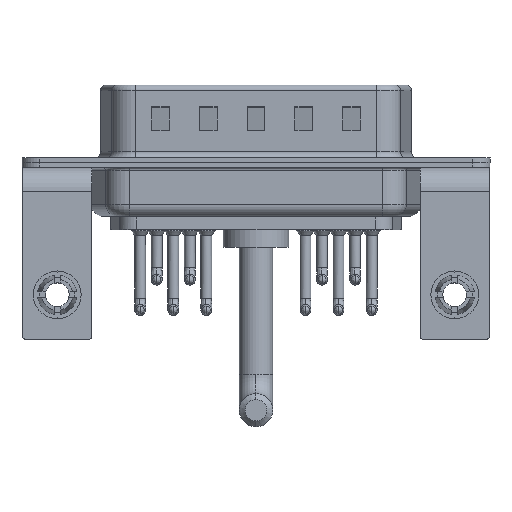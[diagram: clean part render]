
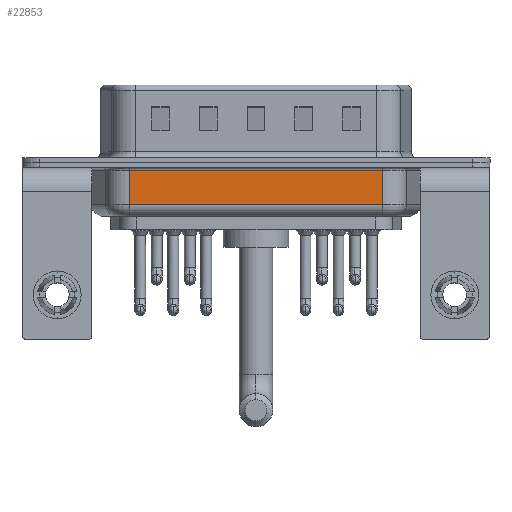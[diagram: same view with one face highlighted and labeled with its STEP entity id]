
A CAD part, front view. The second image highlights one B-rep face of the part: STEP entity #22853.
In plain terms, the highlighted planar face has unit normal (0, -1, 0).
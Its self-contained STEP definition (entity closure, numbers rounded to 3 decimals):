
#396 = DIRECTION ( 'NONE',  ( 0., 0., 1. ) ) ;
#649 = CARTESIAN_POINT ( 'NONE',  ( 6.031, -5.35, -4.5 ) ) ;
#786 = EDGE_CURVE ( 'NONE', #24470, #14708, #24488, .T. ) ;
#2434 = ORIENTED_EDGE ( 'NONE', *, *, #786, .F. ) ;
#3555 = ORIENTED_EDGE ( 'NONE', *, *, #17695, .T. ) ;
#3703 = VECTOR ( 'NONE', #5802, 1000. ) ;
#4075 = LINE ( 'NONE', #22612, #17971 ) ;
#4181 = DIRECTION ( 'NONE',  ( 0., 1., 0. ) ) ;
#4306 = FACE_OUTER_BOUND ( 'NONE', #11699, .T. ) ;
#4551 = VERTEX_POINT ( 'NONE', #9557 ) ;
#5802 = DIRECTION ( 'NONE',  ( -1., 0., 0. ) ) ;
#7107 = CARTESIAN_POINT ( 'NONE',  ( 6.031, -5.35, -4.5 ) ) ;
#7892 = CARTESIAN_POINT ( 'NONE',  ( 6.031, -5.35, -3.5 ) ) ;
#8897 = VECTOR ( 'NONE', #10876, 1000. ) ;
#9557 = CARTESIAN_POINT ( 'NONE',  ( 27.269, -5.35, -3.5 ) ) ;
#9853 = DIRECTION ( 'NONE',  ( 0., 0., 1. ) ) ;
#10165 = CARTESIAN_POINT ( 'NONE',  ( 27.269, -5.35, -0.65 ) ) ;
#10876 = DIRECTION ( 'NONE',  ( 0., 0., 1. ) ) ;
#11699 = EDGE_LOOP ( 'NONE', ( #2434, #3555, #16457, #16517 ) ) ;
#12101 = VERTEX_POINT ( 'NONE', #10165 ) ;
#13299 = DIRECTION ( 'NONE',  ( 1., 0., 0. ) ) ;
#13680 = VECTOR ( 'NONE', #13299, 1000. ) ;
#14000 = EDGE_CURVE ( 'NONE', #4551, #12101, #4075, .T. ) ;
#14708 = VERTEX_POINT ( 'NONE', #21811 ) ;
#15340 = CARTESIAN_POINT ( 'NONE',  ( 6.031, -5.35, -0.65 ) ) ;
#16457 = ORIENTED_EDGE ( 'NONE', *, *, #14000, .T. ) ;
#16517 = ORIENTED_EDGE ( 'NONE', *, *, #20115, .T. ) ;
#16945 = CARTESIAN_POINT ( 'NONE',  ( 6.031, -5.35, -3.5 ) ) ;
#17050 = LINE ( 'NONE', #7892, #13680 ) ;
#17084 = LINE ( 'NONE', #15340, #3703 ) ;
#17695 = EDGE_CURVE ( 'NONE', #24470, #4551, #17050, .T. ) ;
#17971 = VECTOR ( 'NONE', #9853, 1000. ) ;
#20115 = EDGE_CURVE ( 'NONE', #12101, #14708, #17084, .T. ) ;
#21811 = CARTESIAN_POINT ( 'NONE',  ( 6.031, -5.35, -0.65 ) ) ;
#22612 = CARTESIAN_POINT ( 'NONE',  ( 27.269, -5.35, -4.5 ) ) ;
#22853 = ADVANCED_FACE ( 'NONE', ( #4306 ), #23829, .F. ) ;
#23396 = AXIS2_PLACEMENT_3D ( 'NONE', #649, #4181, #396 ) ;
#23829 = PLANE ( 'NONE',  #23396 ) ;
#24470 = VERTEX_POINT ( 'NONE', #16945 ) ;
#24488 = LINE ( 'NONE', #7107, #8897 ) ;
